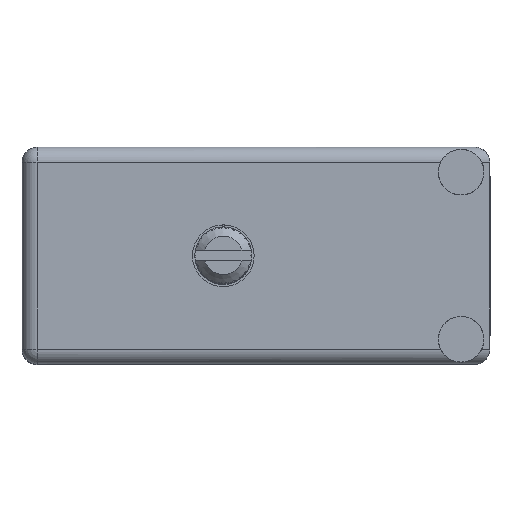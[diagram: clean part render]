
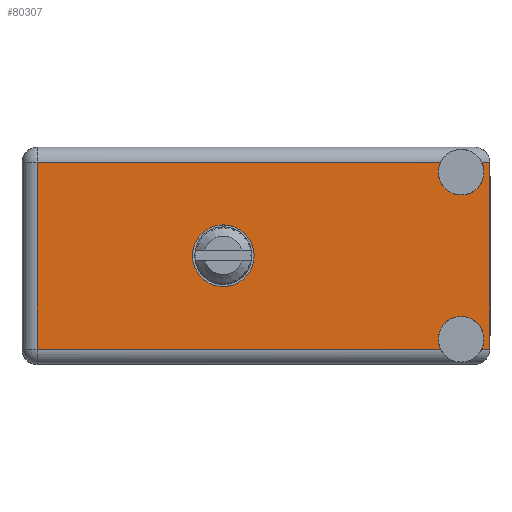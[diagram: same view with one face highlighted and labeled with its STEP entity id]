
A CAD part, top view. The second image highlights one B-rep face of the part: STEP entity #80307.
In plain terms, the highlighted face is planar.
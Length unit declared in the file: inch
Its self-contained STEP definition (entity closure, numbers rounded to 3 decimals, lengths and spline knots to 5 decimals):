
#1751 = DIRECTION ( 'NONE',  ( 0., 0., 1. ) ) ;
#2054 = CIRCLE ( 'NONE', #46010, 0.075 ) ;
#3249 = VECTOR ( 'NONE', #3465, 39.37008 ) ;
#3465 = DIRECTION ( 'NONE',  ( -1., 0., 0. ) ) ;
#4671 = DIRECTION ( 'NONE',  ( 0., 0., 1. ) ) ;
#7744 = CARTESIAN_POINT ( 'NONE',  ( 0.6625, 0.906, -0.459 ) ) ;
#8443 = CARTESIAN_POINT ( 'NONE',  ( 1.445, 0.906, -0.6325 ) ) ;
#8658 = LINE ( 'NONE', #25348, #171971 ) ;
#13154 = ORIENTED_EDGE ( 'NONE', *, *, #28282, .F. ) ;
#14539 = ORIENTED_EDGE ( 'NONE', *, *, #116629, .T. ) ;
#17645 = DIRECTION ( 'NONE',  ( 0., 1., 0. ) ) ;
#19272 = DIRECTION ( 'NONE',  ( 0., 1., 0. ) ) ;
#22840 = DIRECTION ( 'NONE',  ( 1., 0., 0. ) ) ;
#23639 = ORIENTED_EDGE ( 'NONE', *, *, #177833, .F. ) ;
#25348 = CARTESIAN_POINT ( 'NONE',  ( 0.05, 0.906, -0.715 ) ) ;
#26728 = CARTESIAN_POINT ( 'NONE',  ( 0.05, 0.906, -0.05 ) ) ;
#28282 = EDGE_CURVE ( 'NONE', #34190, #81647, #87213, .T. ) ;
#31904 = CIRCLE ( 'NONE', #94640, 0.1015 ) ;
#33335 = EDGE_CURVE ( 'NONE', #91454, #60578, #189205, .T. ) ;
#34188 = VERTEX_POINT ( 'NONE', #137290 ) ;
#34190 = VERTEX_POINT ( 'NONE', #62588 ) ;
#35204 = CARTESIAN_POINT ( 'NONE',  ( 1.445, 0.906, -0.6325 ) ) ;
#41806 = AXIS2_PLACEMENT_3D ( 'NONE', #35204, #95179, #66612 ) ;
#46010 = AXIS2_PLACEMENT_3D ( 'NONE', #98746, #96797, #82032 ) ;
#46422 = VECTOR ( 'NONE', #22840, 39.37008 ) ;
#52146 = EDGE_CURVE ( 'NONE', #81647, #107989, #2054, .T. ) ;
#53245 = DIRECTION ( 'NONE',  ( 1., 0., 0. ) ) ;
#54422 = ORIENTED_EDGE ( 'NONE', *, *, #167204, .T. ) ;
#54477 = CARTESIAN_POINT ( 'NONE',  ( 0., 0.906, -0.715 ) ) ;
#58326 = VERTEX_POINT ( 'NONE', #26728 ) ;
#58400 = CARTESIAN_POINT ( 'NONE',  ( 1.51259, 0.906, -0.665 ) ) ;
#59951 = DIRECTION ( 'NONE',  ( 0., 1., 0. ) ) ;
#60578 = VERTEX_POINT ( 'NONE', #107366 ) ;
#62588 = CARTESIAN_POINT ( 'NONE',  ( 1.51259, 0.906, -0.05 ) ) ;
#62639 = CARTESIAN_POINT ( 'NONE',  ( 0.05, 0.906, -0.665 ) ) ;
#64451 = CARTESIAN_POINT ( 'NONE',  ( 1.539, 0.906, -0.05 ) ) ;
#66612 = DIRECTION ( 'NONE',  ( 0., 0., 1. ) ) ;
#66742 = VERTEX_POINT ( 'NONE', #7744 ) ;
#67000 = VERTEX_POINT ( 'NONE', #93868 ) ;
#67390 = ORIENTED_EDGE ( 'NONE', *, *, #52146, .F. ) ;
#68862 = CIRCLE ( 'NONE', #93996, 0.1015 ) ;
#69218 = FACE_OUTER_BOUND ( 'NONE', #84076, .T. ) ;
#70582 = DIRECTION ( 'NONE',  ( 0., 0., 1. ) ) ;
#70986 = ORIENTED_EDGE ( 'NONE', *, *, #101365, .T. ) ;
#73732 = VERTEX_POINT ( 'NONE', #58400 ) ;
#75669 = CIRCLE ( 'NONE', #132247, 0.075 ) ;
#76233 = VECTOR ( 'NONE', #4671, 39.37008 ) ;
#77786 = AXIS2_PLACEMENT_3D ( 'NONE', #108767, #19272, #104913 ) ;
#80307 = ADVANCED_FACE ( 'NONE', ( #83973, #69218 ), #189087, .T. ) ;
#81647 = VERTEX_POINT ( 'NONE', #99834 ) ;
#82032 = DIRECTION ( 'NONE',  ( 0., 0., 1. ) ) ;
#83973 = FACE_BOUND ( 'NONE', #173687, .T. ) ;
#84076 = EDGE_LOOP ( 'NONE', ( #54422, #67390, #13154, #140587, #101125, #92302, #183579, #180254, #14539, #70986 ) ) ;
#84158 = DIRECTION ( 'NONE',  ( 0., 0., 1. ) ) ;
#85623 = CARTESIAN_POINT ( 'NONE',  ( 0., 0.906, -0.665 ) ) ;
#87213 = CIRCLE ( 'NONE', #77786, 0.075 ) ;
#89308 = CARTESIAN_POINT ( 'NONE',  ( 0.6625, 0.906, -0.256 ) ) ;
#89325 = LINE ( 'NONE', #123683, #76233 ) ;
#91454 = VERTEX_POINT ( 'NONE', #105427 ) ;
#92302 = ORIENTED_EDGE ( 'NONE', *, *, #116265, .T. ) ;
#93868 = CARTESIAN_POINT ( 'NONE',  ( 1.539, 0.906, -0.665 ) ) ;
#93996 = AXIS2_PLACEMENT_3D ( 'NONE', #137549, #59951, #106158 ) ;
#94640 = AXIS2_PLACEMENT_3D ( 'NONE', #121740, #148293, #1751 ) ;
#95179 = DIRECTION ( 'NONE',  ( 0., 1., 0. ) ) ;
#96797 = DIRECTION ( 'NONE',  ( 0., 1., 0. ) ) ;
#98746 = CARTESIAN_POINT ( 'NONE',  ( 1.445, 0.906, -0.0825 ) ) ;
#99834 = CARTESIAN_POINT ( 'NONE',  ( 1.445, 0.906, -0.1575 ) ) ;
#100516 = LINE ( 'NONE', #64451, #46422 ) ;
#101125 = ORIENTED_EDGE ( 'NONE', *, *, #128828, .F. ) ;
#101365 = EDGE_CURVE ( 'NONE', #181204, #58326, #8658, .T. ) ;
#104111 = LINE ( 'NONE', #192519, #3249 ) ;
#104268 = LINE ( 'NONE', #85623, #163421 ) ;
#104867 = EDGE_CURVE ( 'NONE', #34190, #34188, #140759, .T. ) ;
#104913 = DIRECTION ( 'NONE',  ( 0., 0., 1. ) ) ;
#105427 = CARTESIAN_POINT ( 'NONE',  ( 1.37741, 0.906, -0.665 ) ) ;
#106158 = DIRECTION ( 'NONE',  ( 0., 0., 1. ) ) ;
#107366 = CARTESIAN_POINT ( 'NONE',  ( 1.445, 0.906, -0.5575 ) ) ;
#107989 = VERTEX_POINT ( 'NONE', #174968 ) ;
#108456 = ORIENTED_EDGE ( 'NONE', *, *, #120939, .F. ) ;
#108767 = CARTESIAN_POINT ( 'NONE',  ( 1.445, 0.906, -0.0825 ) ) ;
#110289 = AXIS2_PLACEMENT_3D ( 'NONE', #54477, #174360, #175327 ) ;
#116265 = EDGE_CURVE ( 'NONE', #67000, #73732, #104111, .T. ) ;
#116629 = EDGE_CURVE ( 'NONE', #91454, #181204, #104268, .T. ) ;
#119183 = EDGE_CURVE ( 'NONE', #60578, #73732, #75669, .T. ) ;
#120939 = EDGE_CURVE ( 'NONE', #149533, #66742, #31904, .T. ) ;
#121740 = CARTESIAN_POINT ( 'NONE',  ( 0.6625, 0.906, -0.3575 ) ) ;
#123683 = CARTESIAN_POINT ( 'NONE',  ( 1.539, 0.906, 0. ) ) ;
#128828 = EDGE_CURVE ( 'NONE', #67000, #34188, #89325, .T. ) ;
#132247 = AXIS2_PLACEMENT_3D ( 'NONE', #8443, #17645, #84158 ) ;
#137290 = CARTESIAN_POINT ( 'NONE',  ( 1.539, 0.906, -0.05 ) ) ;
#137549 = CARTESIAN_POINT ( 'NONE',  ( 0.6625, 0.906, -0.3575 ) ) ;
#140587 = ORIENTED_EDGE ( 'NONE', *, *, #104867, .T. ) ;
#140759 = LINE ( 'NONE', #187865, #140816 ) ;
#140816 = VECTOR ( 'NONE', #53245, 39.37008 ) ;
#148293 = DIRECTION ( 'NONE',  ( 0., 1., 0. ) ) ;
#149533 = VERTEX_POINT ( 'NONE', #89308 ) ;
#163421 = VECTOR ( 'NONE', #190750, 39.37008 ) ;
#167204 = EDGE_CURVE ( 'NONE', #58326, #107989, #100516, .T. ) ;
#171971 = VECTOR ( 'NONE', #70582, 39.37008 ) ;
#173687 = EDGE_LOOP ( 'NONE', ( #108456, #23639 ) ) ;
#174360 = DIRECTION ( 'NONE',  ( 0., 1., 0. ) ) ;
#174968 = CARTESIAN_POINT ( 'NONE',  ( 1.37741, 0.906, -0.05 ) ) ;
#175327 = DIRECTION ( 'NONE',  ( 0., 0., 1. ) ) ;
#177833 = EDGE_CURVE ( 'NONE', #66742, #149533, #68862, .T. ) ;
#180254 = ORIENTED_EDGE ( 'NONE', *, *, #33335, .F. ) ;
#181204 = VERTEX_POINT ( 'NONE', #62639 ) ;
#183579 = ORIENTED_EDGE ( 'NONE', *, *, #119183, .F. ) ;
#187865 = CARTESIAN_POINT ( 'NONE',  ( 1.539, 0.906, -0.05 ) ) ;
#189087 = PLANE ( 'NONE',  #110289 ) ;
#189205 = CIRCLE ( 'NONE', #41806, 0.075 ) ;
#190750 = DIRECTION ( 'NONE',  ( -1., 0., 0. ) ) ;
#192519 = CARTESIAN_POINT ( 'NONE',  ( 0., 0.906, -0.665 ) ) ;
